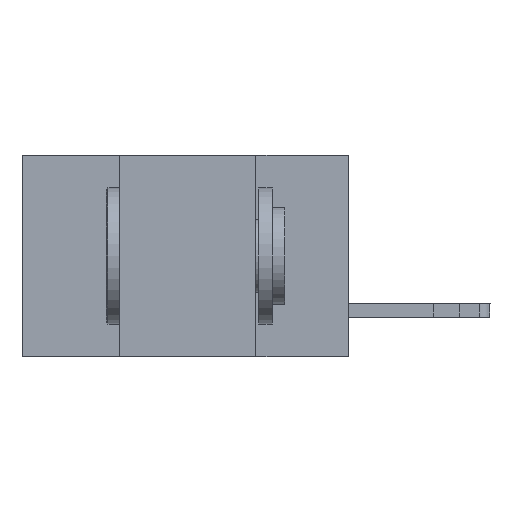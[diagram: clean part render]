
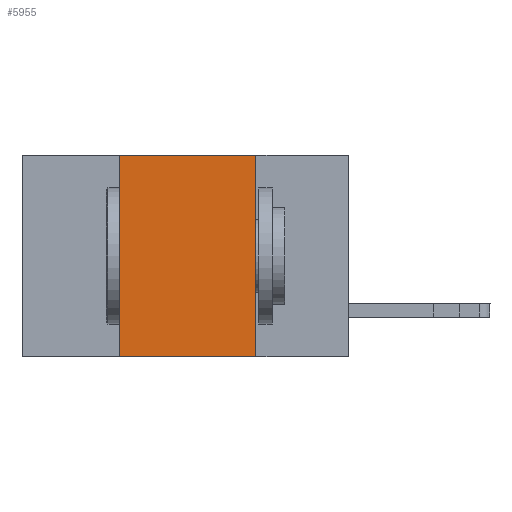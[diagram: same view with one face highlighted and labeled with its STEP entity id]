
A CAD part, left-side view. The second image highlights one B-rep face of the part: STEP entity #5955.
In plain terms, the highlighted planar face has unit normal (-1, 0, 0).
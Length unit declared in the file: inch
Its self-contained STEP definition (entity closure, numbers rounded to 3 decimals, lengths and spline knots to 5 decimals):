
#57 = VECTOR ( 'NONE', #1605, 39.37008 ) ;
#220 = EDGE_CURVE ( 'NONE', #5159, #14062, #7854, .T. ) ;
#1100 = ORIENTED_EDGE ( 'NONE', *, *, #6558, .T. ) ;
#1605 = DIRECTION ( 'NONE',  ( 0., 0., -1. ) ) ;
#2388 = DIRECTION ( 'NONE',  ( 0., 0., 1. ) ) ;
#2993 = AXIS2_PLACEMENT_3D ( 'NONE', #11512, #3928, #8793 ) ;
#3001 = VECTOR ( 'NONE', #14237, 39.37008 ) ;
#3928 = DIRECTION ( 'NONE',  ( 1., 0., 0. ) ) ;
#4104 = LINE ( 'NONE', #14157, #3001 ) ;
#4227 = CARTESIAN_POINT ( 'NONE',  ( 0., 0.17, -0.37 ) ) ;
#5005 = FACE_OUTER_BOUND ( 'NONE', #5437, .T. ) ;
#5061 = CARTESIAN_POINT ( 'NONE',  ( 0., 0.17, -0.37 ) ) ;
#5159 = VERTEX_POINT ( 'NONE', #13723 ) ;
#5437 = EDGE_LOOP ( 'NONE', ( #15066, #14776, #16081, #1100 ) ) ;
#5610 = EDGE_CURVE ( 'NONE', #10546, #5159, #15305, .T. ) ;
#5955 = ADVANCED_FACE ( 'NONE', ( #5005 ), #13973, .F. ) ;
#6558 = EDGE_CURVE ( 'NONE', #13145, #14062, #4104, .T. ) ;
#6660 = VECTOR ( 'NONE', #12835, 39.37008 ) ;
#7854 = LINE ( 'NONE', #4227, #57 ) ;
#8793 = DIRECTION ( 'NONE',  ( 0., 0., -1. ) ) ;
#8794 = LINE ( 'NONE', #11105, #8852 ) ;
#8852 = VECTOR ( 'NONE', #2388, 39.37008 ) ;
#10546 = VERTEX_POINT ( 'NONE', #11218 ) ;
#11105 = CARTESIAN_POINT ( 'NONE',  ( 0., 0.42, -0.37 ) ) ;
#11218 = CARTESIAN_POINT ( 'NONE',  ( 0., 0.42, 0. ) ) ;
#11512 = CARTESIAN_POINT ( 'NONE',  ( 0., 0.6, 0. ) ) ;
#12601 = CARTESIAN_POINT ( 'NONE',  ( 0., 0.42, -0.37 ) ) ;
#12835 = DIRECTION ( 'NONE',  ( 0., -1., 0. ) ) ;
#13145 = VERTEX_POINT ( 'NONE', #12601 ) ;
#13510 = EDGE_CURVE ( 'NONE', #13145, #10546, #8794, .T. ) ;
#13723 = CARTESIAN_POINT ( 'NONE',  ( 0., 0.17, 0. ) ) ;
#13841 = CARTESIAN_POINT ( 'NONE',  ( 0., 0.6, 0. ) ) ;
#13973 = PLANE ( 'NONE',  #2993 ) ;
#14062 = VERTEX_POINT ( 'NONE', #5061 ) ;
#14157 = CARTESIAN_POINT ( 'NONE',  ( 0., 0.6, -0.37 ) ) ;
#14237 = DIRECTION ( 'NONE',  ( 0., -1., 0. ) ) ;
#14776 = ORIENTED_EDGE ( 'NONE', *, *, #5610, .F. ) ;
#15066 = ORIENTED_EDGE ( 'NONE', *, *, #220, .F. ) ;
#15305 = LINE ( 'NONE', #13841, #6660 ) ;
#16081 = ORIENTED_EDGE ( 'NONE', *, *, #13510, .F. ) ;
